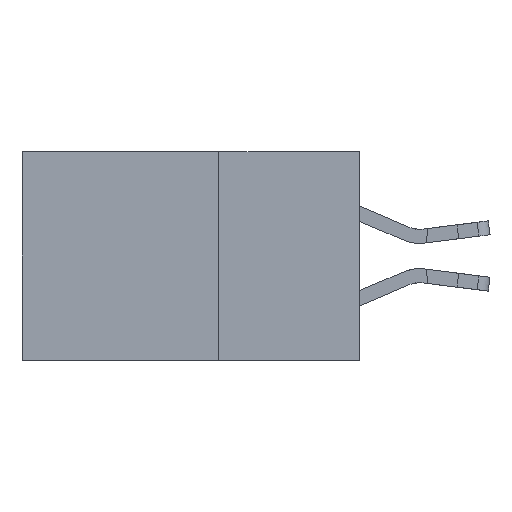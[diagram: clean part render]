
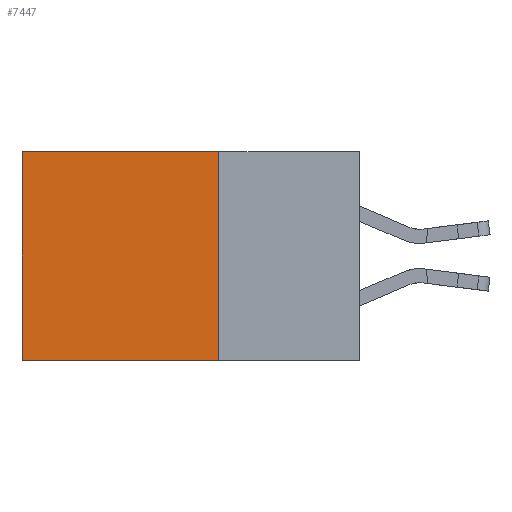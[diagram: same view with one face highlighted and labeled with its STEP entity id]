
A CAD part, left-side view. The second image highlights one B-rep face of the part: STEP entity #7447.
In plain terms, the highlighted planar face has unit normal (-1, 0, 0).
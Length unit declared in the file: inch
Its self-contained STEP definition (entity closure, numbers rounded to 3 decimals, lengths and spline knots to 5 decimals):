
#347 = CARTESIAN_POINT ( 'NONE',  ( 0.2875, 0.25, 0. ) ) ;
#1538 = DIRECTION ( 'NONE',  ( 0., 1., 0. ) ) ;
#2298 = CARTESIAN_POINT ( 'NONE',  ( 0.2875, 0.6, 0. ) ) ;
#3268 = CARTESIAN_POINT ( 'NONE',  ( 0.2875, 0.6, 0. ) ) ;
#3441 = EDGE_CURVE ( 'NONE', #15537, #5264, #15130, .T. ) ;
#3468 = EDGE_LOOP ( 'NONE', ( #6847, #9065, #8240, #12772 ) ) ;
#4441 = LINE ( 'NONE', #15821, #15490 ) ;
#4584 = EDGE_CURVE ( 'NONE', #12111, #15537, #4441, .T. ) ;
#4758 = CARTESIAN_POINT ( 'NONE',  ( 0.2875, 0.25, -0.37 ) ) ;
#5264 = VERTEX_POINT ( 'NONE', #16039 ) ;
#6847 = ORIENTED_EDGE ( 'NONE', *, *, #11087, .T. ) ;
#7323 = CARTESIAN_POINT ( 'NONE',  ( 0.2875, 0.25, 0. ) ) ;
#7447 = ADVANCED_FACE ( 'NONE', ( #9093 ), #14937, .F. ) ;
#7508 = LINE ( 'NONE', #14887, #10855 ) ;
#7656 = VECTOR ( 'NONE', #15964, 39.37008 ) ;
#8240 = ORIENTED_EDGE ( 'NONE', *, *, #4584, .F. ) ;
#8722 = DIRECTION ( 'NONE',  ( 0., 0., -1. ) ) ;
#9065 = ORIENTED_EDGE ( 'NONE', *, *, #3441, .F. ) ;
#9093 = FACE_OUTER_BOUND ( 'NONE', #3468, .T. ) ;
#9525 = DIRECTION ( 'NONE',  ( 0., 0., -1. ) ) ;
#9670 = LINE ( 'NONE', #2298, #7656 ) ;
#9713 = VERTEX_POINT ( 'NONE', #3268 ) ;
#10755 = AXIS2_PLACEMENT_3D ( 'NONE', #7323, #14101, #8722 ) ;
#10855 = VECTOR ( 'NONE', #13663, 39.37008 ) ;
#11087 = EDGE_CURVE ( 'NONE', #9713, #5264, #9670, .T. ) ;
#12111 = VERTEX_POINT ( 'NONE', #347 ) ;
#12772 = ORIENTED_EDGE ( 'NONE', *, *, #12969, .T. ) ;
#12969 = EDGE_CURVE ( 'NONE', #12111, #9713, #7508, .T. ) ;
#13025 = VECTOR ( 'NONE', #1538, 39.37008 ) ;
#13187 = CARTESIAN_POINT ( 'NONE',  ( 0.2875, 0.25, -0.37 ) ) ;
#13663 = DIRECTION ( 'NONE',  ( 0., 1., 0. ) ) ;
#14101 = DIRECTION ( 'NONE',  ( 1., 0., 0. ) ) ;
#14887 = CARTESIAN_POINT ( 'NONE',  ( 0.2875, 0.25, 0. ) ) ;
#14937 = PLANE ( 'NONE',  #10755 ) ;
#15130 = LINE ( 'NONE', #4758, #13025 ) ;
#15490 = VECTOR ( 'NONE', #9525, 39.37008 ) ;
#15537 = VERTEX_POINT ( 'NONE', #13187 ) ;
#15821 = CARTESIAN_POINT ( 'NONE',  ( 0.2875, 0.25, 0. ) ) ;
#15964 = DIRECTION ( 'NONE',  ( 0., 0., -1. ) ) ;
#16039 = CARTESIAN_POINT ( 'NONE',  ( 0.2875, 0.6, -0.37 ) ) ;
